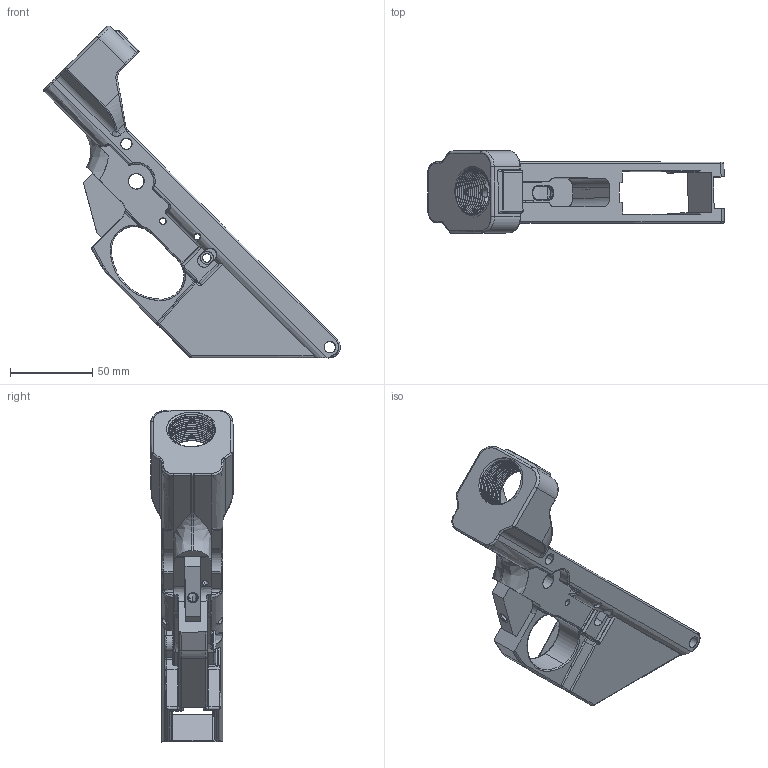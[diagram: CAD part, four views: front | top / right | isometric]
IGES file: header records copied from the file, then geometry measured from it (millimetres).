
Start section: SolidWorks IGES file using analytic representation for surfaces
Global section: file name: Abraxas_JT_AR-10_V1.IGS; native system: SolidWorks 2015; preprocessor: SolidWorks 2015; author: WarFairy; date: 150522.140759; units: inch
Bounding box: 180.12 x 50.23 x 201.59 mm (x, y, z)
Surface area: 65958.9 mm2 (no closed solid volume)
Topology: 0 solids, 0 shells, 475 faces, 6294 edges, 6278 vertices
Faces by surface type: bspline 247, revolution 228
